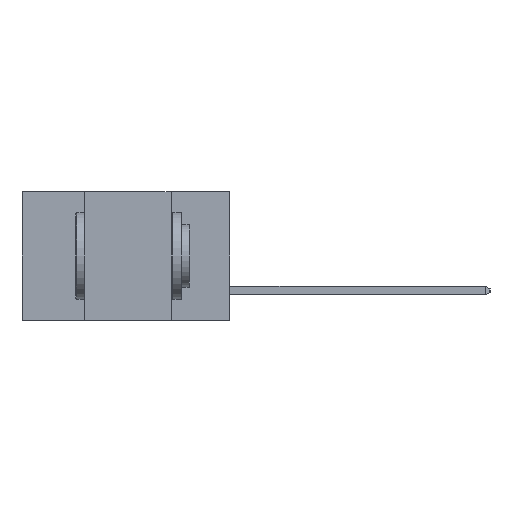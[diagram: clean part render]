
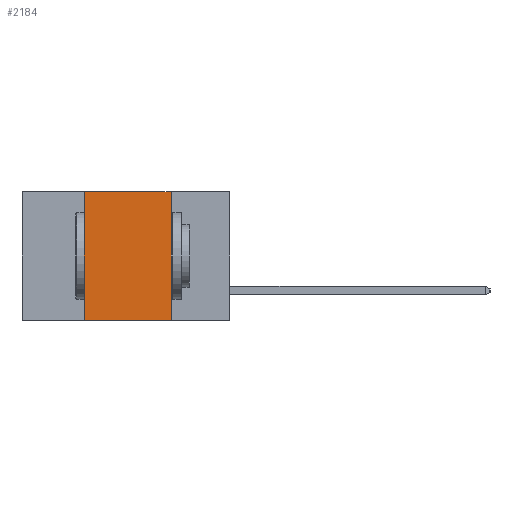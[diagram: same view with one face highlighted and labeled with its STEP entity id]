
A CAD part, left-side view. The second image highlights one B-rep face of the part: STEP entity #2184.
In plain terms, the highlighted planar face has unit normal (-1, 0, 0).
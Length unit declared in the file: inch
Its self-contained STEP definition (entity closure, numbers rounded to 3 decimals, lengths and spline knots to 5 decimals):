
#340 = CARTESIAN_POINT ( 'NONE',  ( 0., 0.17, 0. ) ) ;
#2184 = ADVANCED_FACE ( 'NONE', ( #21577 ), #16721, .F. ) ;
#2578 = VERTEX_POINT ( 'NONE', #11209 ) ;
#3861 = AXIS2_PLACEMENT_3D ( 'NONE', #8294, #8267, #5531 ) ;
#4465 = CARTESIAN_POINT ( 'NONE',  ( 0., 0.17, 0. ) ) ;
#4480 = VERTEX_POINT ( 'NONE', #4465 ) ;
#5531 = DIRECTION ( 'NONE',  ( 0., 0., -1. ) ) ;
#5797 = LINE ( 'NONE', #340, #22016 ) ;
#8044 = LINE ( 'NONE', #20542, #8630 ) ;
#8267 = DIRECTION ( 'NONE',  ( 1., 0., 0. ) ) ;
#8294 = CARTESIAN_POINT ( 'NONE',  ( 0., 0.6, 0. ) ) ;
#8630 = VECTOR ( 'NONE', #11520, 39.37008 ) ;
#10011 = ORIENTED_EDGE ( 'NONE', *, *, #12654, .F. ) ;
#10254 = CARTESIAN_POINT ( 'NONE',  ( 0., 0.17, -0.37 ) ) ;
#10528 = ORIENTED_EDGE ( 'NONE', *, *, #14789, .F. ) ;
#10614 = ORIENTED_EDGE ( 'NONE', *, *, #21015, .F. ) ;
#10712 = LINE ( 'NONE', #19573, #19756 ) ;
#11086 = ORIENTED_EDGE ( 'NONE', *, *, #15101, .T. ) ;
#11209 = CARTESIAN_POINT ( 'NONE',  ( 0., 0.42, -0.37 ) ) ;
#11520 = DIRECTION ( 'NONE',  ( 0., -1., 0. ) ) ;
#12047 = VERTEX_POINT ( 'NONE', #19186 ) ;
#12654 = EDGE_CURVE ( 'NONE', #4480, #20375, #5797, .T. ) ;
#13318 = VECTOR ( 'NONE', #22808, 39.37008 ) ;
#14789 = EDGE_CURVE ( 'NONE', #12047, #4480, #10712, .T. ) ;
#15101 = EDGE_CURVE ( 'NONE', #2578, #20375, #8044, .T. ) ;
#16721 = PLANE ( 'NONE',  #3861 ) ;
#18095 = LINE ( 'NONE', #21076, #13318 ) ;
#19186 = CARTESIAN_POINT ( 'NONE',  ( 0., 0.42, 0. ) ) ;
#19573 = CARTESIAN_POINT ( 'NONE',  ( 0., 0.6, 0. ) ) ;
#19715 = EDGE_LOOP ( 'NONE', ( #10011, #10528, #10614, #11086 ) ) ;
#19756 = VECTOR ( 'NONE', #21308, 39.37008 ) ;
#20375 = VERTEX_POINT ( 'NONE', #10254 ) ;
#20542 = CARTESIAN_POINT ( 'NONE',  ( 0., 0.6, -0.37 ) ) ;
#21015 = EDGE_CURVE ( 'NONE', #2578, #12047, #18095, .T. ) ;
#21076 = CARTESIAN_POINT ( 'NONE',  ( 0., 0.42, 0. ) ) ;
#21308 = DIRECTION ( 'NONE',  ( 0., -1., 0. ) ) ;
#21577 = FACE_OUTER_BOUND ( 'NONE', #19715, .T. ) ;
#22016 = VECTOR ( 'NONE', #22539, 39.37008 ) ;
#22539 = DIRECTION ( 'NONE',  ( 0., 0., -1. ) ) ;
#22808 = DIRECTION ( 'NONE',  ( 0., 0., 1. ) ) ;
